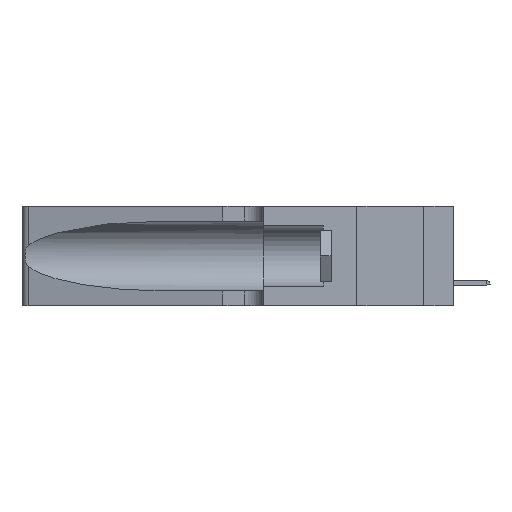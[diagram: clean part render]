
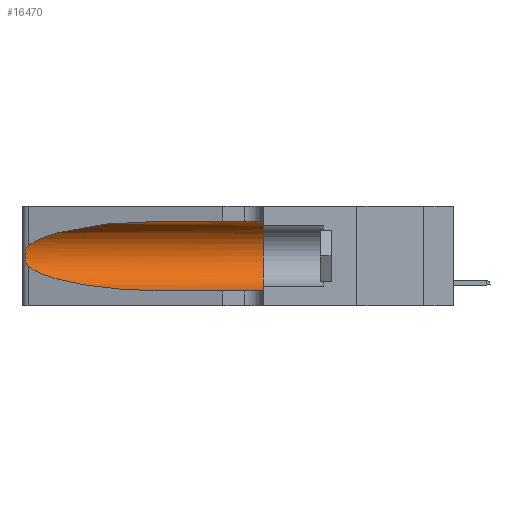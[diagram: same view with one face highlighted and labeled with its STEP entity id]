
A CAD part, left-side view. The second image highlights one B-rep face of the part: STEP entity #16470.
In plain terms, the highlighted cylindrical face has radius 3.308 mm (diameter 6.617 mm), a partial arc.
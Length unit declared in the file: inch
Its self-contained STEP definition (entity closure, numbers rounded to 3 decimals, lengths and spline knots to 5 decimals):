
#442 = DIRECTION ( 'NONE',  ( 0., -1., 0. ) ) ;
#863 = CARTESIAN_POINT ( 'NONE',  ( 0.25639, 1.23184, 0.21858 ) ) ;
#1064 = CARTESIAN_POINT ( 'NONE',  ( 0.26017, 1.23833, 0.17102 ) ) ;
#1636 = CARTESIAN_POINT ( 'NONE',  ( 0.1305, 0.35, 0.05475 ) ) ;
#3622 = ORIENTED_EDGE ( 'NONE', *, *, #38651, .T. ) ;
#4191 = VERTEX_POINT ( 'NONE', #36803 ) ;
#4219 = CARTESIAN_POINT ( 'NONE',  ( 0.25555, 1.22993, 0.14849 ) ) ;
#4388 = CARTESIAN_POINT ( 'NONE',  ( 0.25487, 1.22718, 0.14631 ) ) ;
#4731 =( BOUNDED_CURVE ( )  B_SPLINE_CURVE ( 3, ( #4388, #36410, #32862, #23446 ),
 .UNSPECIFIED., .F., .T. ) 
 B_SPLINE_CURVE_WITH_KNOTS ( ( 4, 4 ),
 ( 3.44316, 4.71239 ),
 .UNSPECIFIED. ) 
 CURVE ( )  GEOMETRIC_REPRESENTATION_ITEM ( )  RATIONAL_B_SPLINE_CURVE ( ( 1., 0.87, 0.87, 1. ) ) 
 REPRESENTATION_ITEM ( '' )  );
#5847 = CARTESIAN_POINT ( 'NONE',  ( 0.2373, 1.15595, 0.28018 ) ) ;
#6167 = LINE ( 'NONE', #37981, #37484 ) ;
#7373 = CARTESIAN_POINT ( 'NONE',  ( 0.25789, 1.23486, 0.15765 ) ) ;
#9162 = VERTEX_POINT ( 'NONE', #19984 ) ;
#9577 = EDGE_CURVE ( 'NONE', #29155, #35800, #4731, .T. ) ;
#9683 = CYLINDRICAL_SURFACE ( 'NONE', #25030, 0.13025 ) ;
#9875 = AXIS2_PLACEMENT_3D ( 'NONE', #11663, #37191, #17304 ) ;
#10099 = CARTESIAN_POINT ( 'NONE',  ( 0.25787, 1.23484, 0.2124 ) ) ;
#10249 = ORIENTED_EDGE ( 'NONE', *, *, #34630, .F. ) ;
#11663 = CARTESIAN_POINT ( 'NONE',  ( 0.1305, 0.35, 0.185 ) ) ;
#12140 = CARTESIAN_POINT ( 'NONE',  ( 0.1305, 0.72297, 0.31525 ) ) ;
#12343 = CARTESIAN_POINT ( 'NONE',  ( 0.1305, 1.61858, 0.31525 ) ) ;
#13211 = CIRCLE ( 'NONE', #9875, 0.13025 ) ;
#13768 = EDGE_CURVE ( 'NONE', #4191, #21554, #17560, .T. ) ;
#13838 = CARTESIAN_POINT ( 'NONE',  ( 0.26018, 1.23835, 0.19895 ) ) ;
#16159 = FACE_OUTER_BOUND ( 'NONE', #34703, .T. ) ;
#16470 = ADVANCED_FACE ( 'NONE', ( #16159 ), #9683, .F. ) ;
#16567 = CARTESIAN_POINT ( 'NONE',  ( 0.26075, 1.23896, 0.19203 ) ) ;
#16779 = CARTESIAN_POINT ( 'NONE',  ( 0.25555, 1.22994, 0.2215 ) ) ;
#17201 = VERTEX_POINT ( 'NONE', #1636 ) ;
#17304 = DIRECTION ( 'NONE',  ( 0., 0., 1. ) ) ;
#17560 =( BOUNDED_CURVE ( )  B_SPLINE_CURVE ( 3, ( #12140, #37667, #5847, #31600 ),
 .UNSPECIFIED., .F., .T. ) 
 B_SPLINE_CURVE_WITH_KNOTS ( ( 4, 4 ),
 ( 1.5708, 2.84003 ),
 .UNSPECIFIED. ) 
 CURVE ( )  GEOMETRIC_REPRESENTATION_ITEM ( )  RATIONAL_B_SPLINE_CURVE ( ( 1., 0.87, 0.87, 1. ) ) 
 REPRESENTATION_ITEM ( '' )  );
#18476 = ORIENTED_EDGE ( 'NONE', *, *, #30226, .F. ) ;
#18528 = DIRECTION ( 'NONE',  ( 0., -1., 0. ) ) ;
#19984 = CARTESIAN_POINT ( 'NONE',  ( 0.1305, 0.35, 0.31525 ) ) ;
#21554 = VERTEX_POINT ( 'NONE', #31302 ) ;
#22449 = DIRECTION ( 'NONE',  ( 0., 0., -1. ) ) ;
#22865 = CARTESIAN_POINT ( 'NONE',  ( 0.25854, 1.2359, 0.20912 ) ) ;
#23101 = ORIENTED_EDGE ( 'NONE', *, *, #37680, .T. ) ;
#23268 = CARTESIAN_POINT ( 'NONE',  ( 0.25856, 1.23593, 0.16098 ) ) ;
#23446 = CARTESIAN_POINT ( 'NONE',  ( 0.1305, 0.72297, 0.05475 ) ) ;
#25030 = AXIS2_PLACEMENT_3D ( 'NONE', #25169, #442, #22449 ) ;
#25169 = CARTESIAN_POINT ( 'NONE',  ( 0.1305, 1.61858, 0.185 ) ) ;
#28451 = VECTOR ( 'NONE', #34736, 39.37008 ) ;
#28532 = ORIENTED_EDGE ( 'NONE', *, *, #13768, .T. ) ;
#29155 = VERTEX_POINT ( 'NONE', #35340 ) ;
#29353 = CARTESIAN_POINT ( 'NONE',  ( 0.26075, 1.23896, 0.178 ) ) ;
#29770 = CARTESIAN_POINT ( 'NONE',  ( 0.25487, 1.22718, 0.14631 ) ) ;
#30226 = EDGE_CURVE ( 'NONE', #4191, #9162, #34524, .T. ) ;
#31302 = CARTESIAN_POINT ( 'NONE',  ( 0.25487, 1.22718, 0.22369 ) ) ;
#31600 = CARTESIAN_POINT ( 'NONE',  ( 0.25487, 1.22718, 0.22369 ) ) ;
#32862 = CARTESIAN_POINT ( 'NONE',  ( 0.18966, 0.96281, 0.05475 ) ) ;
#32889 = CARTESIAN_POINT ( 'NONE',  ( 0.25639, 1.23186, 0.15144 ) ) ;
#34524 = LINE ( 'NONE', #12343, #28451 ) ;
#34630 = EDGE_CURVE ( 'NONE', #9162, #17201, #13211, .T. ) ;
#34703 = EDGE_LOOP ( 'NONE', ( #28532, #3622, #38733, #23101, #10249, #18476 ) ) ;
#34736 = DIRECTION ( 'NONE',  ( 0., -1., 0. ) ) ;
#35340 = CARTESIAN_POINT ( 'NONE',  ( 0.25487, 1.22718, 0.14631 ) ) ;
#35800 = VERTEX_POINT ( 'NONE', #37401 ) ;
#36410 = CARTESIAN_POINT ( 'NONE',  ( 0.2373, 1.15595, 0.08982 ) ) ;
#36504 = B_SPLINE_CURVE_WITH_KNOTS ( 'NONE', 3,
 ( #38773, #16779, #863, #10099, #22865, #13838, #16567, #29353, #1064, #23268, #7373, #32889, #4219, #29770 ),
 .UNSPECIFIED., .F., .F.,
 ( 4, 2, 2, 2, 2, 2, 4 ),
 ( 0., 0.00027, 0.00053, 0.00107, 0.0016, 0.00187, 0.00214 ),
 .UNSPECIFIED. ) ;
#36803 = CARTESIAN_POINT ( 'NONE',  ( 0.1305, 0.72297, 0.31525 ) ) ;
#37191 = DIRECTION ( 'NONE',  ( 0., 1., 0. ) ) ;
#37401 = CARTESIAN_POINT ( 'NONE',  ( 0.1305, 0.72297, 0.05475 ) ) ;
#37484 = VECTOR ( 'NONE', #18528, 39.37008 ) ;
#37667 = CARTESIAN_POINT ( 'NONE',  ( 0.18966, 0.96281, 0.31525 ) ) ;
#37680 = EDGE_CURVE ( 'NONE', #35800, #17201, #6167, .T. ) ;
#37981 = CARTESIAN_POINT ( 'NONE',  ( 0.1305, 1.61858, 0.05475 ) ) ;
#38651 = EDGE_CURVE ( 'NONE', #21554, #29155, #36504, .T. ) ;
#38733 = ORIENTED_EDGE ( 'NONE', *, *, #9577, .T. ) ;
#38773 = CARTESIAN_POINT ( 'NONE',  ( 0.25487, 1.22718, 0.22369 ) ) ;
